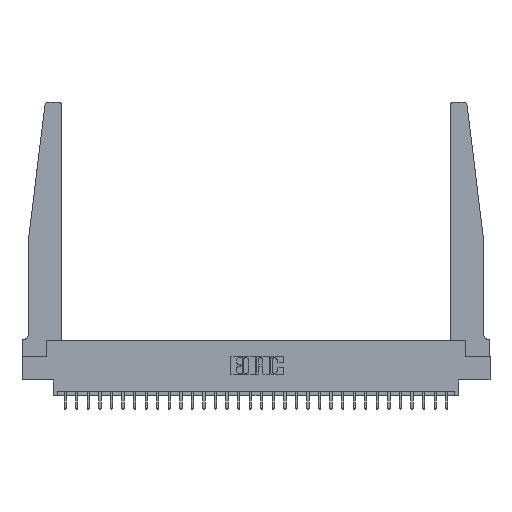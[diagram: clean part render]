
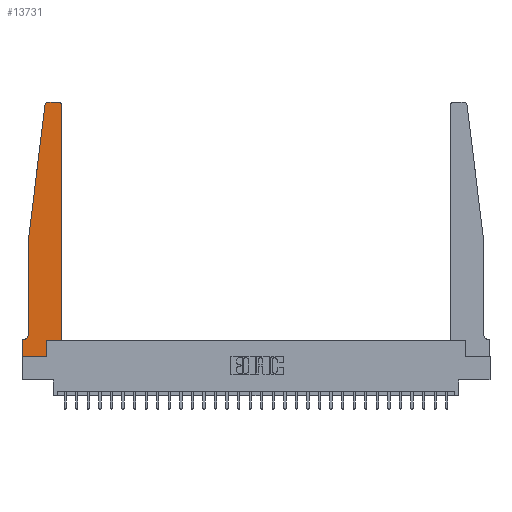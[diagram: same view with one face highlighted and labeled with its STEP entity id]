
A CAD part, top view. The second image highlights one B-rep face of the part: STEP entity #13731.
In plain terms, the highlighted planar face has unit normal (0, 0, 1).
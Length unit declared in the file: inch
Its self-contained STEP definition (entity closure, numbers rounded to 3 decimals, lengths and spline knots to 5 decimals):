
#112 = DIRECTION ( 'NONE',  ( 0., 0., -1. ) ) ;
#334 = EDGE_CURVE ( 'NONE', #8372, #5460, #28035, .T. ) ;
#343 = CARTESIAN_POINT ( 'NONE',  ( 0.395, 2.75, 0.37 ) ) ;
#653 = EDGE_CURVE ( 'NONE', #2737, #24116, #20682, .T. ) ;
#1628 = VERTEX_POINT ( 'NONE', #22103 ) ;
#1697 = DIRECTION ( 'NONE',  ( 0., -1., 0. ) ) ;
#1804 = AXIS2_PLACEMENT_3D ( 'NONE', #6748, #9584, #9527 ) ;
#1882 = EDGE_CURVE ( 'NONE', #14881, #8372, #20658, .T. ) ;
#1938 = DIRECTION ( 'NONE',  ( 0., 0., 1. ) ) ;
#2091 = LINE ( 'NONE', #4659, #13079 ) ;
#2172 = CARTESIAN_POINT ( 'NONE',  ( 0.425, 0.18, 0.37 ) ) ;
#2201 = DIRECTION ( 'NONE',  ( -1., 0., 0. ) ) ;
#2737 = VERTEX_POINT ( 'NONE', #17370 ) ;
#3071 = EDGE_CURVE ( 'NONE', #3719, #1628, #25989, .T. ) ;
#3138 = CARTESIAN_POINT ( 'NONE',  ( 0.065, 1.25, 0.37 ) ) ;
#3672 = ORIENTED_EDGE ( 'NONE', *, *, #11586, .T. ) ;
#3714 = VERTEX_POINT ( 'NONE', #23328 ) ;
#3719 = VERTEX_POINT ( 'NONE', #27588 ) ;
#3885 = VERTEX_POINT ( 'NONE', #23775 ) ;
#4207 = DIRECTION ( 'NONE',  ( -1., 0., 0. ) ) ;
#4659 = CARTESIAN_POINT ( 'NONE',  ( 0.425, 0.18, 0.37 ) ) ;
#4899 = CARTESIAN_POINT ( 'NONE',  ( 0., 0., 0.37 ) ) ;
#5000 = CARTESIAN_POINT ( 'NONE',  ( 0., 0.1875, 0.37 ) ) ;
#5460 = VERTEX_POINT ( 'NONE', #343 ) ;
#5993 = LINE ( 'NONE', #3138, #6670 ) ;
#6065 = ORIENTED_EDGE ( 'NONE', *, *, #27943, .T. ) ;
#6079 = LINE ( 'NONE', #15276, #24135 ) ;
#6225 = EDGE_CURVE ( 'NONE', #20626, #2737, #5993, .T. ) ;
#6670 = VECTOR ( 'NONE', #20641, 39.37008 ) ;
#6748 = CARTESIAN_POINT ( 'NONE',  ( 0.395, 2.72, 0.37 ) ) ;
#6896 = DIRECTION ( 'NONE',  ( 1., 0., 0. ) ) ;
#6975 = AXIS2_PLACEMENT_3D ( 'NONE', #24281, #11199, #26428 ) ;
#7998 = CARTESIAN_POINT ( 'NONE',  ( 0.24675, 2.72367, 0.37 ) ) ;
#8372 = VERTEX_POINT ( 'NONE', #18044 ) ;
#9056 = VECTOR ( 'NONE', #25174, 39.37008 ) ;
#9079 = VECTOR ( 'NONE', #1697, 39.37008 ) ;
#9527 = DIRECTION ( 'NONE',  ( 1., 0., 0. ) ) ;
#9584 = DIRECTION ( 'NONE',  ( 0., 0., 1. ) ) ;
#10465 = ORIENTED_EDGE ( 'NONE', *, *, #13309, .T. ) ;
#10654 = VECTOR ( 'NONE', #18892, 39.37008 ) ;
#10963 = CARTESIAN_POINT ( 'NONE',  ( 0.015, 0.1875, 0.37 ) ) ;
#11199 = DIRECTION ( 'NONE',  ( 0., 0., 1. ) ) ;
#11508 = EDGE_CURVE ( 'NONE', #5460, #3714, #6079, .T. ) ;
#11586 = EDGE_CURVE ( 'NONE', #3714, #20626, #11855, .T. ) ;
#11855 = CIRCLE ( 'NONE', #6975, 0.03 ) ;
#11943 = CARTESIAN_POINT ( 'NONE',  ( 0., 0., 0.37 ) ) ;
#12047 = DIRECTION ( 'NONE',  ( 1., 0., 0. ) ) ;
#12641 = CARTESIAN_POINT ( 'NONE',  ( 0.065, 1.25, 0.37 ) ) ;
#12779 = VECTOR ( 'NONE', #4207, 39.37008 ) ;
#12886 = PLANE ( 'NONE',  #15743 ) ;
#13079 = VECTOR ( 'NONE', #6896, 39.37008 ) ;
#13287 = CARTESIAN_POINT ( 'NONE',  ( 0.015, 0.2375, 0.37 ) ) ;
#13309 = EDGE_CURVE ( 'NONE', #19205, #3719, #13539, .T. ) ;
#13539 = LINE ( 'NONE', #4899, #24456 ) ;
#13731 = ADVANCED_FACE ( 'NONE', ( #14827 ), #12886, .T. ) ;
#14413 = VECTOR ( 'NONE', #12047, 39.37008 ) ;
#14452 = ORIENTED_EDGE ( 'NONE', *, *, #653, .T. ) ;
#14827 = FACE_OUTER_BOUND ( 'NONE', #25360, .T. ) ;
#14836 = EDGE_CURVE ( 'NONE', #27535, #19205, #15808, .T. ) ;
#14881 = VERTEX_POINT ( 'NONE', #2172 ) ;
#14983 = ORIENTED_EDGE ( 'NONE', *, *, #11508, .T. ) ;
#15018 = ORIENTED_EDGE ( 'NONE', *, *, #334, .T. ) ;
#15276 = CARTESIAN_POINT ( 'NONE',  ( 0.25, 2.75, 0.37 ) ) ;
#15433 = DIRECTION ( 'NONE',  ( -1., 0., 0. ) ) ;
#15743 = AXIS2_PLACEMENT_3D ( 'NONE', #27981, #1938, #17235 ) ;
#15808 = LINE ( 'NONE', #28112, #12779 ) ;
#16397 = ORIENTED_EDGE ( 'NONE', *, *, #1882, .T. ) ;
#16438 = ORIENTED_EDGE ( 'NONE', *, *, #20909, .T. ) ;
#16658 = CARTESIAN_POINT ( 'NONE',  ( 0.2605, 0.18, 0.37 ) ) ;
#17232 = AXIS2_PLACEMENT_3D ( 'NONE', #13287, #112, #15433 ) ;
#17235 = DIRECTION ( 'NONE',  ( 1., 0., 0. ) ) ;
#17370 = CARTESIAN_POINT ( 'NONE',  ( 0.065, 1.25, 0.37 ) ) ;
#18044 = CARTESIAN_POINT ( 'NONE',  ( 0.425, 2.72, 0.37 ) ) ;
#18139 = CIRCLE ( 'NONE', #17232, 0.05 ) ;
#18154 = ORIENTED_EDGE ( 'NONE', *, *, #3071, .T. ) ;
#18161 = DIRECTION ( 'NONE',  ( 0., -1., 0. ) ) ;
#18892 = DIRECTION ( 'NONE',  ( 0., 1., 0. ) ) ;
#19205 = VERTEX_POINT ( 'NONE', #5000 ) ;
#20626 = VERTEX_POINT ( 'NONE', #7998 ) ;
#20641 = DIRECTION ( 'NONE',  ( -0.122, -0.992, 0. ) ) ;
#20658 = LINE ( 'NONE', #22974, #9056 ) ;
#20682 = LINE ( 'NONE', #12641, #9079 ) ;
#20909 = EDGE_CURVE ( 'NONE', #24116, #27535, #18139, .T. ) ;
#21491 = ORIENTED_EDGE ( 'NONE', *, *, #27606, .T. ) ;
#22103 = CARTESIAN_POINT ( 'NONE',  ( 0.2605, 0., 0.37 ) ) ;
#22974 = CARTESIAN_POINT ( 'NONE',  ( 0.425, 0.18, 0.37 ) ) ;
#23328 = CARTESIAN_POINT ( 'NONE',  ( 0.27653, 2.75, 0.37 ) ) ;
#23775 = CARTESIAN_POINT ( 'NONE',  ( 0.2605, 0.18, 0.37 ) ) ;
#24116 = VERTEX_POINT ( 'NONE', #25278 ) ;
#24135 = VECTOR ( 'NONE', #2201, 39.37008 ) ;
#24281 = CARTESIAN_POINT ( 'NONE',  ( 0.27653, 2.72, 0.37 ) ) ;
#24364 = ORIENTED_EDGE ( 'NONE', *, *, #6225, .T. ) ;
#24456 = VECTOR ( 'NONE', #18161, 39.37008 ) ;
#24530 = ORIENTED_EDGE ( 'NONE', *, *, #14836, .T. ) ;
#25174 = DIRECTION ( 'NONE',  ( 0., 1., 0. ) ) ;
#25278 = CARTESIAN_POINT ( 'NONE',  ( 0.065, 0.2375, 0.37 ) ) ;
#25360 = EDGE_LOOP ( 'NONE', ( #14983, #3672, #24364, #14452, #16438, #24530, #10465, #18154, #6065, #21491, #16397, #15018 ) ) ;
#25989 = LINE ( 'NONE', #11943, #14413 ) ;
#26428 = DIRECTION ( 'NONE',  ( 1., 0., 0. ) ) ;
#27293 = LINE ( 'NONE', #16658, #10654 ) ;
#27535 = VERTEX_POINT ( 'NONE', #10963 ) ;
#27588 = CARTESIAN_POINT ( 'NONE',  ( 0., 0., 0.37 ) ) ;
#27606 = EDGE_CURVE ( 'NONE', #3885, #14881, #2091, .T. ) ;
#27943 = EDGE_CURVE ( 'NONE', #1628, #3885, #27293, .T. ) ;
#27981 = CARTESIAN_POINT ( 'NONE',  ( 0., 0.1875, 0.37 ) ) ;
#28035 = CIRCLE ( 'NONE', #1804, 0.03 ) ;
#28112 = CARTESIAN_POINT ( 'NONE',  ( 0.065, 0.1875, 0.37 ) ) ;
